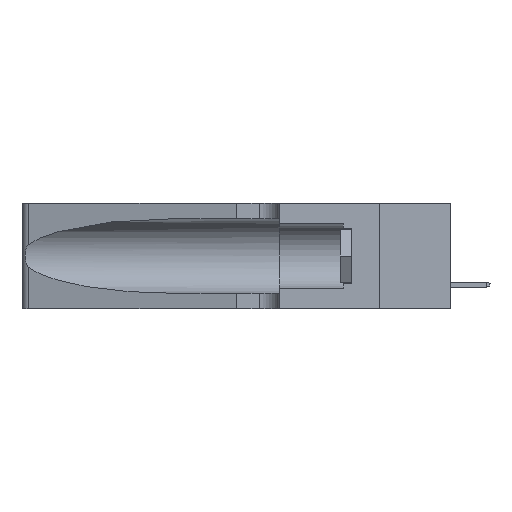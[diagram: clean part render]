
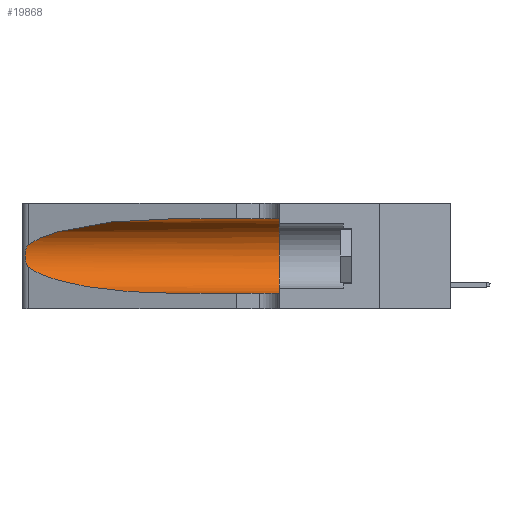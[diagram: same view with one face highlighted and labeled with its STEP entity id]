
A CAD part, left-side view. The second image highlights one B-rep face of the part: STEP entity #19868.
In plain terms, the highlighted cylindrical face has radius 3.308 mm (diameter 6.617 mm), a partial arc.
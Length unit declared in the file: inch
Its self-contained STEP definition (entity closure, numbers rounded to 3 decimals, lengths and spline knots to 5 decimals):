
#179 = CARTESIAN_POINT ( 'NONE',  ( 0.1305, 0.35, 0.185 ) ) ;
#610 = LINE ( 'NONE', #11259, #26973 ) ;
#648 = ORIENTED_EDGE ( 'NONE', *, *, #34117, .F. ) ;
#1967 = CARTESIAN_POINT ( 'NONE',  ( 0.1305, 1.61858, 0.31525 ) ) ;
#2183 = CARTESIAN_POINT ( 'NONE',  ( 0.25639, 1.23184, 0.21858 ) ) ;
#2688 = CARTESIAN_POINT ( 'NONE',  ( 0.18966, 0.96281, 0.31525 ) ) ;
#2728 = VERTEX_POINT ( 'NONE', #20124 ) ;
#3529 = DIRECTION ( 'NONE',  ( 0., 0., -1. ) ) ;
#4798 =( BOUNDED_CURVE ( )  B_SPLINE_CURVE ( 3, ( #10716, #2688, #13664, #23965 ),
 .UNSPECIFIED., .F., .T. ) 
 B_SPLINE_CURVE_WITH_KNOTS ( ( 4, 4 ),
 ( 1.5708, 2.84003 ),
 .UNSPECIFIED. ) 
 CURVE ( )  GEOMETRIC_REPRESENTATION_ITEM ( )  RATIONAL_B_SPLINE_CURVE ( ( 1., 0.87, 0.87, 1. ) ) 
 REPRESENTATION_ITEM ( '' )  );
#5137 = CARTESIAN_POINT ( 'NONE',  ( 0.26017, 1.23833, 0.17102 ) ) ;
#6102 = VERTEX_POINT ( 'NONE', #24281 ) ;
#6166 = DIRECTION ( 'NONE',  ( 0., -1., 0. ) ) ;
#7245 = VERTEX_POINT ( 'NONE', #13789 ) ;
#7427 = CARTESIAN_POINT ( 'NONE',  ( 0.25555, 1.22994, 0.2215 ) ) ;
#8657 = ORIENTED_EDGE ( 'NONE', *, *, #30104, .F. ) ;
#8735 = ORIENTED_EDGE ( 'NONE', *, *, #9626, .T. ) ;
#9483 = FACE_OUTER_BOUND ( 'NONE', #27281, .T. ) ;
#9626 = EDGE_CURVE ( 'NONE', #7245, #20926, #610, .T. ) ;
#9700 = CARTESIAN_POINT ( 'NONE',  ( 0.26018, 1.23835, 0.19895 ) ) ;
#10206 = CARTESIAN_POINT ( 'NONE',  ( 0.25789, 1.23486, 0.15765 ) ) ;
#10388 = CARTESIAN_POINT ( 'NONE',  ( 0.26075, 1.23896, 0.178 ) ) ;
#10716 = CARTESIAN_POINT ( 'NONE',  ( 0.1305, 0.72297, 0.31525 ) ) ;
#11259 = CARTESIAN_POINT ( 'NONE',  ( 0.1305, 1.61858, 0.05475 ) ) ;
#13664 = CARTESIAN_POINT ( 'NONE',  ( 0.2373, 1.15595, 0.28018 ) ) ;
#13789 = CARTESIAN_POINT ( 'NONE',  ( 0.1305, 0.72297, 0.05475 ) ) ;
#14353 = CYLINDRICAL_SURFACE ( 'NONE', #22715, 0.13025 ) ;
#15315 = CARTESIAN_POINT ( 'NONE',  ( 0.1305, 0.35, 0.05475 ) ) ;
#17391 = CIRCLE ( 'NONE', #21841, 0.13025 ) ;
#17445 = VERTEX_POINT ( 'NONE', #25869 ) ;
#17548 = CARTESIAN_POINT ( 'NONE',  ( 0.2373, 1.15595, 0.08982 ) ) ;
#18044 = CARTESIAN_POINT ( 'NONE',  ( 0.26075, 1.23896, 0.19203 ) ) ;
#18056 = CARTESIAN_POINT ( 'NONE',  ( 0.18966, 0.96281, 0.05475 ) ) ;
#18791 = EDGE_CURVE ( 'NONE', #17445, #23764, #4798, .T. ) ;
#19556 = EDGE_CURVE ( 'NONE', #23764, #6102, #21526, .T. ) ;
#19868 = ADVANCED_FACE ( 'NONE', ( #9483 ), #14353, .F. ) ;
#20124 = CARTESIAN_POINT ( 'NONE',  ( 0.1305, 0.35, 0.31525 ) ) ;
#20409 = ORIENTED_EDGE ( 'NONE', *, *, #19556, .T. ) ;
#20926 = VERTEX_POINT ( 'NONE', #15315 ) ;
#21526 = B_SPLINE_CURVE_WITH_KNOTS ( 'NONE', 3,
 ( #23629, #7427, #2183, #25711, #29017, #9700, #18044, #10388, #5137, #28673, #10206, #30959, #34090, #25547 ),
 .UNSPECIFIED., .F., .F.,
 ( 4, 2, 2, 2, 2, 2, 4 ),
 ( 0., 0.00027, 0.00053, 0.00107, 0.0016, 0.00187, 0.00214 ),
 .UNSPECIFIED. ) ;
#21841 = AXIS2_PLACEMENT_3D ( 'NONE', #179, #32613, #24587 ) ;
#21891 = DIRECTION ( 'NONE',  ( 0., -1., 0. ) ) ;
#22715 = AXIS2_PLACEMENT_3D ( 'NONE', #27398, #6166, #3529 ) ;
#22769 = CARTESIAN_POINT ( 'NONE',  ( 0.25487, 1.22718, 0.14631 ) ) ;
#23629 = CARTESIAN_POINT ( 'NONE',  ( 0.25487, 1.22718, 0.22369 ) ) ;
#23764 = VERTEX_POINT ( 'NONE', #31740 ) ;
#23965 = CARTESIAN_POINT ( 'NONE',  ( 0.25487, 1.22718, 0.22369 ) ) ;
#24281 = CARTESIAN_POINT ( 'NONE',  ( 0.25487, 1.22718, 0.14631 ) ) ;
#24587 = DIRECTION ( 'NONE',  ( 0., 0., 1. ) ) ;
#25547 = CARTESIAN_POINT ( 'NONE',  ( 0.25487, 1.22718, 0.14631 ) ) ;
#25703 = ORIENTED_EDGE ( 'NONE', *, *, #31387, .T. ) ;
#25711 = CARTESIAN_POINT ( 'NONE',  ( 0.25787, 1.23484, 0.2124 ) ) ;
#25847 = LINE ( 'NONE', #1967, #31417 ) ;
#25869 = CARTESIAN_POINT ( 'NONE',  ( 0.1305, 0.72297, 0.31525 ) ) ;
#26013 = DIRECTION ( 'NONE',  ( 0., -1., 0. ) ) ;
#26497 = ORIENTED_EDGE ( 'NONE', *, *, #18791, .T. ) ;
#26973 = VECTOR ( 'NONE', #21891, 39.37008 ) ;
#27281 = EDGE_LOOP ( 'NONE', ( #26497, #20409, #25703, #8735, #648, #8657 ) ) ;
#27398 = CARTESIAN_POINT ( 'NONE',  ( 0.1305, 1.61858, 0.185 ) ) ;
#27487 =( BOUNDED_CURVE ( )  B_SPLINE_CURVE ( 3, ( #22769, #17548, #18056, #28165 ),
 .UNSPECIFIED., .F., .T. ) 
 B_SPLINE_CURVE_WITH_KNOTS ( ( 4, 4 ),
 ( 3.44316, 4.71239 ),
 .UNSPECIFIED. ) 
 CURVE ( )  GEOMETRIC_REPRESENTATION_ITEM ( )  RATIONAL_B_SPLINE_CURVE ( ( 1., 0.87, 0.87, 1. ) ) 
 REPRESENTATION_ITEM ( '' )  );
#28165 = CARTESIAN_POINT ( 'NONE',  ( 0.1305, 0.72297, 0.05475 ) ) ;
#28673 = CARTESIAN_POINT ( 'NONE',  ( 0.25856, 1.23593, 0.16098 ) ) ;
#29017 = CARTESIAN_POINT ( 'NONE',  ( 0.25854, 1.2359, 0.20912 ) ) ;
#30104 = EDGE_CURVE ( 'NONE', #17445, #2728, #25847, .T. ) ;
#30959 = CARTESIAN_POINT ( 'NONE',  ( 0.25639, 1.23186, 0.15144 ) ) ;
#31387 = EDGE_CURVE ( 'NONE', #6102, #7245, #27487, .T. ) ;
#31417 = VECTOR ( 'NONE', #26013, 39.37008 ) ;
#31740 = CARTESIAN_POINT ( 'NONE',  ( 0.25487, 1.22718, 0.22369 ) ) ;
#32613 = DIRECTION ( 'NONE',  ( 0., 1., 0. ) ) ;
#34090 = CARTESIAN_POINT ( 'NONE',  ( 0.25555, 1.22993, 0.14849 ) ) ;
#34117 = EDGE_CURVE ( 'NONE', #2728, #20926, #17391, .T. ) ;
